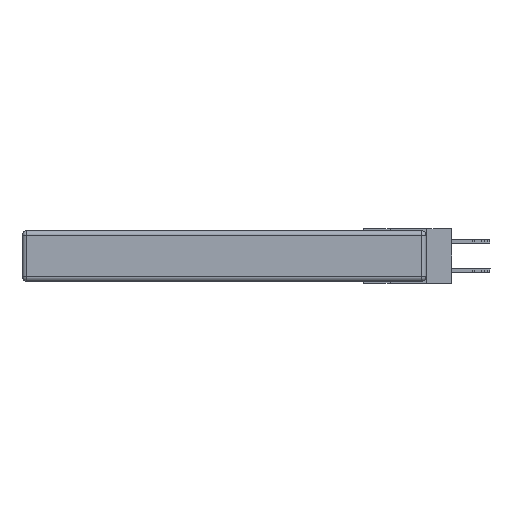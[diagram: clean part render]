
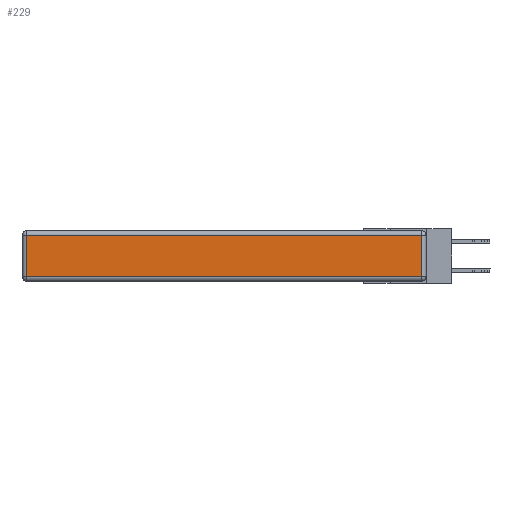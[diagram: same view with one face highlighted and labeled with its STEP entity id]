
A CAD part, left-side view. The second image highlights one B-rep face of the part: STEP entity #229.
In plain terms, the highlighted planar face has unit normal (-1, 0, 0).
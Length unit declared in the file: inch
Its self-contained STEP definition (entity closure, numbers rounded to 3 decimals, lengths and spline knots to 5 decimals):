
#116 = PLANE ( 'NONE',  #7262 ) ;
#229 = ADVANCED_FACE ( 'NONE', ( #5729 ), #116, .T. ) ;
#813 = EDGE_CURVE ( 'NONE', #4084, #21825, #32122, .T. ) ;
#1506 = EDGE_CURVE ( 'NONE', #21825, #32184, #11507, .T. ) ;
#2710 = EDGE_CURVE ( 'NONE', #21311, #4084, #23180, .T. ) ;
#4084 = VERTEX_POINT ( 'NONE', #16671 ) ;
#4409 = VECTOR ( 'NONE', #7801, 39.37008 ) ;
#5729 = FACE_OUTER_BOUND ( 'NONE', #9701, .T. ) ;
#7067 = CARTESIAN_POINT ( 'NONE',  ( 0., 2.72, -0.313 ) ) ;
#7262 = AXIS2_PLACEMENT_3D ( 'NONE', #8111, #16150, #10677 ) ;
#7801 = DIRECTION ( 'NONE',  ( 0., 0., -1. ) ) ;
#8111 = CARTESIAN_POINT ( 'NONE',  ( 0., 0., -0.343 ) ) ;
#8537 = ORIENTED_EDGE ( 'NONE', *, *, #1506, .T. ) ;
#9701 = EDGE_LOOP ( 'NONE', ( #8537, #31145, #12287, #19094 ) ) ;
#10127 = DIRECTION ( 'NONE',  ( 0., -1., 0. ) ) ;
#10677 = DIRECTION ( 'NONE',  ( 0., 0., 1. ) ) ;
#11507 = LINE ( 'NONE', #18083, #12751 ) ;
#12287 = ORIENTED_EDGE ( 'NONE', *, *, #2710, .T. ) ;
#12751 = VECTOR ( 'NONE', #10127, 39.37008 ) ;
#15226 = CARTESIAN_POINT ( 'NONE',  ( 0., 0.03, -0.343 ) ) ;
#16150 = DIRECTION ( 'NONE',  ( -1., 0., 0. ) ) ;
#16487 = CARTESIAN_POINT ( 'NONE',  ( 0., 0.03, -0.03 ) ) ;
#16671 = CARTESIAN_POINT ( 'NONE',  ( 0., 2.72, -0.03 ) ) ;
#18083 = CARTESIAN_POINT ( 'NONE',  ( 0., 0., -0.313 ) ) ;
#19094 = ORIENTED_EDGE ( 'NONE', *, *, #813, .T. ) ;
#21311 = VERTEX_POINT ( 'NONE', #16487 ) ;
#21514 = VECTOR ( 'NONE', #23281, 39.37008 ) ;
#21551 = CARTESIAN_POINT ( 'NONE',  ( 0., 2.72, -0.343 ) ) ;
#21825 = VERTEX_POINT ( 'NONE', #7067 ) ;
#23045 = CARTESIAN_POINT ( 'NONE',  ( 0., 2.75, -0.03 ) ) ;
#23180 = LINE ( 'NONE', #23045, #21514 ) ;
#23281 = DIRECTION ( 'NONE',  ( 0., 1., 0. ) ) ;
#25158 = EDGE_CURVE ( 'NONE', #32184, #21311, #34404, .T. ) ;
#27846 = CARTESIAN_POINT ( 'NONE',  ( 0., 0.03, -0.313 ) ) ;
#28900 = VECTOR ( 'NONE', #29223, 39.37008 ) ;
#29223 = DIRECTION ( 'NONE',  ( 0., 0., 1. ) ) ;
#31145 = ORIENTED_EDGE ( 'NONE', *, *, #25158, .T. ) ;
#32122 = LINE ( 'NONE', #21551, #4409 ) ;
#32184 = VERTEX_POINT ( 'NONE', #27846 ) ;
#34404 = LINE ( 'NONE', #15226, #28900 ) ;
